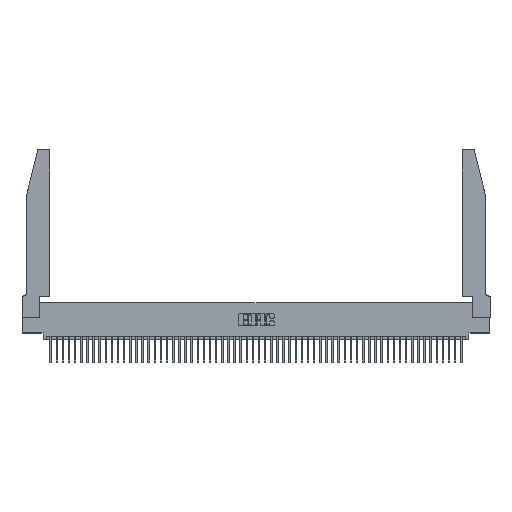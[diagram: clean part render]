
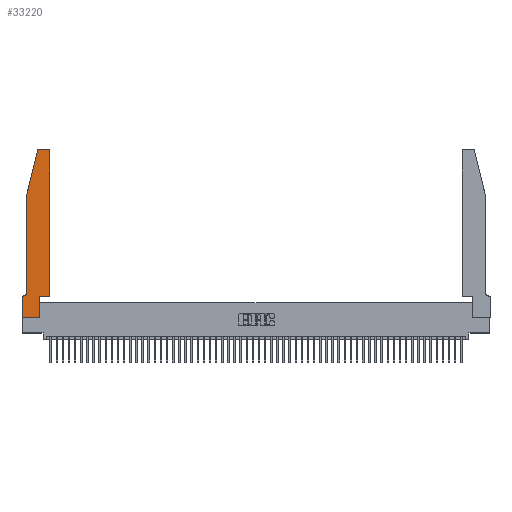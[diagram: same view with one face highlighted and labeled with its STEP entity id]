
A CAD part, top view. The second image highlights one B-rep face of the part: STEP entity #33220.
In plain terms, the highlighted planar face has unit normal (0, 0, 1).
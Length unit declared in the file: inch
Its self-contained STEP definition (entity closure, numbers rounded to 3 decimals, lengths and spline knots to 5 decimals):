
#642 = CARTESIAN_POINT ( 'NONE',  ( 0.0055, 0.35, 0.37 ) ) ;
#745 = DIRECTION ( 'NONE',  ( 1., 0., 0. ) ) ;
#942 = DIRECTION ( 'NONE',  ( 1., 0., 0. ) ) ;
#1453 = LINE ( 'NONE', #50188, #20639 ) ;
#1544 = ORIENTED_EDGE ( 'NONE', *, *, #38323, .T. ) ;
#2189 = LINE ( 'NONE', #50833, #40547 ) ;
#2324 = CARTESIAN_POINT ( 'NONE',  ( 0.4505, 0.35, 0.37 ) ) ;
#3022 = VERTEX_POINT ( 'NONE', #41870 ) ;
#3797 = VERTEX_POINT ( 'NONE', #13078 ) ;
#3801 = EDGE_CURVE ( 'NONE', #34434, #16179, #18151, .T. ) ;
#4313 = EDGE_CURVE ( 'NONE', #48163, #45553, #2189, .T. ) ;
#4921 = VECTOR ( 'NONE', #18659, 39.37008 ) ;
#5252 = ORIENTED_EDGE ( 'NONE', *, *, #15599, .T. ) ;
#5473 = DIRECTION ( 'NONE',  ( 0., 1., 0. ) ) ;
#7422 = DIRECTION ( 'NONE',  ( 1., 0., 0. ) ) ;
#7747 = CARTESIAN_POINT ( 'NONE',  ( 0.0755, 0.35, 0.37 ) ) ;
#8079 = DIRECTION ( 'NONE',  ( 0., -1., 0. ) ) ;
#8099 = CARTESIAN_POINT ( 'NONE',  ( 0.2865, 0.35, 0.37 ) ) ;
#8579 = DIRECTION ( 'NONE',  ( 1., 0., 0. ) ) ;
#8779 = AXIS2_PLACEMENT_3D ( 'NONE', #37542, #29037, #7422 ) ;
#9080 = EDGE_CURVE ( 'NONE', #45112, #23460, #1453, .T. ) ;
#9175 = CARTESIAN_POINT ( 'NONE',  ( 0.4505, 0.35, 0.37 ) ) ;
#9906 = CIRCLE ( 'NONE', #22797, 0.03 ) ;
#10521 = CARTESIAN_POINT ( 'NONE',  ( 0.0755, 0.42, 0.37 ) ) ;
#10666 = DIRECTION ( 'NONE',  ( -1., 0., 0. ) ) ;
#12525 = ORIENTED_EDGE ( 'NONE', *, *, #9080, .T. ) ;
#12746 = DIRECTION ( 'NONE',  ( -1., 0., 0. ) ) ;
#13078 = CARTESIAN_POINT ( 'NONE',  ( 0.284, 2.75, 0.37 ) ) ;
#14056 = EDGE_LOOP ( 'NONE', ( #22752, #22224, #18864, #12525, #54741, #1544, #22053, #42048, #5252, #27890, #18119, #24509 ) ) ;
#14209 = VECTOR ( 'NONE', #53843, 39.37008 ) ;
#15599 = EDGE_CURVE ( 'NONE', #51365, #48163, #52951, .T. ) ;
#16179 = VERTEX_POINT ( 'NONE', #23017 ) ;
#17829 = FACE_OUTER_BOUND ( 'NONE', #14056, .T. ) ;
#18119 = ORIENTED_EDGE ( 'NONE', *, *, #53960, .T. ) ;
#18146 = LINE ( 'NONE', #28355, #14209 ) ;
#18151 = LINE ( 'NONE', #38181, #20811 ) ;
#18659 = DIRECTION ( 'NONE',  ( -1., 0., 0. ) ) ;
#18864 = ORIENTED_EDGE ( 'NONE', *, *, #52085, .T. ) ;
#20639 = VECTOR ( 'NONE', #8079, 39.37008 ) ;
#20811 = VECTOR ( 'NONE', #38524, 39.37008 ) ;
#20855 = CARTESIAN_POINT ( 'NONE',  ( 0.0755, 2., 0.37 ) ) ;
#22053 = ORIENTED_EDGE ( 'NONE', *, *, #3801, .T. ) ;
#22224 = ORIENTED_EDGE ( 'NONE', *, *, #34026, .T. ) ;
#22679 = LINE ( 'NONE', #7747, #45172 ) ;
#22752 = ORIENTED_EDGE ( 'NONE', *, *, #37898, .T. ) ;
#22797 = AXIS2_PLACEMENT_3D ( 'NONE', #46467, #25558, #8579 ) ;
#23017 = CARTESIAN_POINT ( 'NONE',  ( 0., 0., 0.37 ) ) ;
#23460 = VERTEX_POINT ( 'NONE', #10521 ) ;
#24148 = LINE ( 'NONE', #25923, #54594 ) ;
#24509 = ORIENTED_EDGE ( 'NONE', *, *, #50193, .T. ) ;
#25501 = VERTEX_POINT ( 'NONE', #43134 ) ;
#25558 = DIRECTION ( 'NONE',  ( 0., 0., 1. ) ) ;
#25923 = CARTESIAN_POINT ( 'NONE',  ( 0., 0., 0.37 ) ) ;
#26445 = DIRECTION ( 'NONE',  ( 0., 0., 1. ) ) ;
#27445 = CARTESIAN_POINT ( 'NONE',  ( 0.0055, 0.42, 0.37 ) ) ;
#27890 = ORIENTED_EDGE ( 'NONE', *, *, #4313, .T. ) ;
#28355 = CARTESIAN_POINT ( 'NONE',  ( 0.0755, 2., 0.37 ) ) ;
#29037 = DIRECTION ( 'NONE',  ( 0., 0., 1. ) ) ;
#29388 = LINE ( 'NONE', #52648, #4921 ) ;
#31787 = LINE ( 'NONE', #9175, #46322 ) ;
#33220 = ADVANCED_FACE ( 'NONE', ( #17829 ), #41777, .T. ) ;
#33840 = VERTEX_POINT ( 'NONE', #40815 ) ;
#34026 = EDGE_CURVE ( 'NONE', #3797, #3022, #34931, .T. ) ;
#34434 = VERTEX_POINT ( 'NONE', #44560 ) ;
#34931 = CIRCLE ( 'NONE', #36693, 0.03 ) ;
#36577 = DIRECTION ( 'NONE',  ( 0., 1., 0. ) ) ;
#36693 = AXIS2_PLACEMENT_3D ( 'NONE', #43459, #26445, #745 ) ;
#37113 = CARTESIAN_POINT ( 'NONE',  ( 0.2865, 0.35, 0.37 ) ) ;
#37542 = CARTESIAN_POINT ( 'NONE',  ( 0., 0.35, 0.37 ) ) ;
#37898 = EDGE_CURVE ( 'NONE', #33840, #3797, #29388, .T. ) ;
#38181 = CARTESIAN_POINT ( 'NONE',  ( 0., 0., 0.37 ) ) ;
#38323 = EDGE_CURVE ( 'NONE', #38399, #34434, #22679, .T. ) ;
#38399 = VERTEX_POINT ( 'NONE', #642 ) ;
#38524 = DIRECTION ( 'NONE',  ( 0., -1., 0. ) ) ;
#38626 = EDGE_CURVE ( 'NONE', #23460, #38399, #39816, .T. ) ;
#39816 = CIRCLE ( 'NONE', #41901, 0.07 ) ;
#40547 = VECTOR ( 'NONE', #46066, 39.37008 ) ;
#40815 = CARTESIAN_POINT ( 'NONE',  ( 0.4205, 2.75, 0.37 ) ) ;
#41777 = PLANE ( 'NONE',  #8779 ) ;
#41870 = CARTESIAN_POINT ( 'NONE',  ( 0.25487, 2.72718, 0.37 ) ) ;
#41901 = AXIS2_PLACEMENT_3D ( 'NONE', #27445, #44092, #10666 ) ;
#42048 = ORIENTED_EDGE ( 'NONE', *, *, #44140, .T. ) ;
#43134 = CARTESIAN_POINT ( 'NONE',  ( 0.4505, 2.72, 0.37 ) ) ;
#43459 = CARTESIAN_POINT ( 'NONE',  ( 0.284, 2.72, 0.37 ) ) ;
#44092 = DIRECTION ( 'NONE',  ( 0., 0., -1. ) ) ;
#44140 = EDGE_CURVE ( 'NONE', #16179, #51365, #24148, .T. ) ;
#44560 = CARTESIAN_POINT ( 'NONE',  ( 0., 0.35, 0.37 ) ) ;
#45112 = VERTEX_POINT ( 'NONE', #20855 ) ;
#45172 = VECTOR ( 'NONE', #12746, 39.37008 ) ;
#45553 = VERTEX_POINT ( 'NONE', #2324 ) ;
#46066 = DIRECTION ( 'NONE',  ( 1., 0., 0. ) ) ;
#46322 = VECTOR ( 'NONE', #5473, 39.37008 ) ;
#46467 = CARTESIAN_POINT ( 'NONE',  ( 0.4205, 2.72, 0.37 ) ) ;
#48163 = VERTEX_POINT ( 'NONE', #8099 ) ;
#50188 = CARTESIAN_POINT ( 'NONE',  ( 0.0755, 2., 0.37 ) ) ;
#50193 = EDGE_CURVE ( 'NONE', #25501, #33840, #9906, .T. ) ;
#50568 = CARTESIAN_POINT ( 'NONE',  ( 0.2865, 0., 0.37 ) ) ;
#50833 = CARTESIAN_POINT ( 'NONE',  ( 0.4505, 0.35, 0.37 ) ) ;
#51365 = VERTEX_POINT ( 'NONE', #50568 ) ;
#52085 = EDGE_CURVE ( 'NONE', #3022, #45112, #18146, .T. ) ;
#52303 = VECTOR ( 'NONE', #36577, 39.37008 ) ;
#52648 = CARTESIAN_POINT ( 'NONE',  ( 0.2605, 2.75, 0.37 ) ) ;
#52951 = LINE ( 'NONE', #37113, #52303 ) ;
#53843 = DIRECTION ( 'NONE',  ( -0.239, -0.971, 0. ) ) ;
#53960 = EDGE_CURVE ( 'NONE', #45553, #25501, #31787, .T. ) ;
#54594 = VECTOR ( 'NONE', #942, 39.37008 ) ;
#54741 = ORIENTED_EDGE ( 'NONE', *, *, #38626, .T. ) ;
